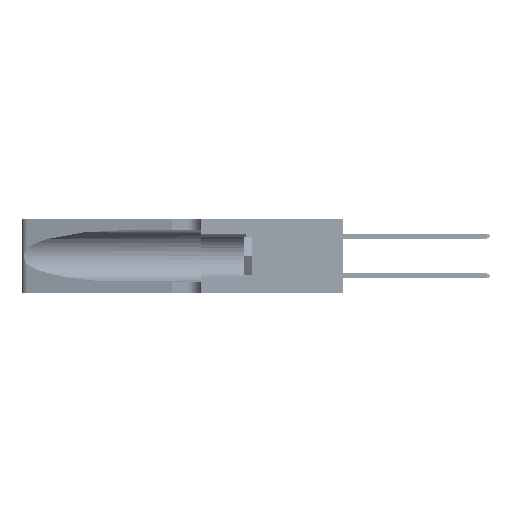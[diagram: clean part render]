
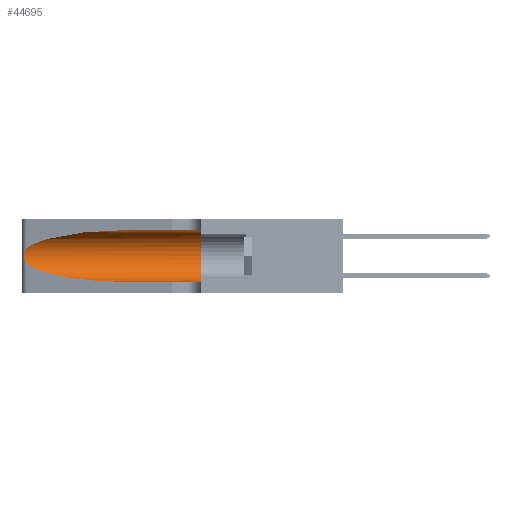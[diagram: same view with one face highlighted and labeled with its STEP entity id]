
A CAD part, left-side view. The second image highlights one B-rep face of the part: STEP entity #44695.
In plain terms, the highlighted cylindrical face has radius 3.308 mm (diameter 6.617 mm), a partial arc.
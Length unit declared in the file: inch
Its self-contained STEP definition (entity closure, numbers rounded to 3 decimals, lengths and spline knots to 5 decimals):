
#1191 = EDGE_CURVE ( 'NONE', #35356, #46719, #9492, .T. ) ;
#1440 = CYLINDRICAL_SURFACE ( 'NONE', #10116, 0.13025 ) ;
#1744 = CARTESIAN_POINT ( 'NONE',  ( 0.25856, 1.23593, 0.16098 ) ) ;
#2813 = FACE_OUTER_BOUND ( 'NONE', #36074, .T. ) ;
#4378 = CARTESIAN_POINT ( 'NONE',  ( 0.1305, 0.72297, 0.05475 ) ) ;
#6072 = ORIENTED_EDGE ( 'NONE', *, *, #26586, .T. ) ;
#6073 = CARTESIAN_POINT ( 'NONE',  ( 0.25639, 1.23186, 0.15144 ) ) ;
#6747 = CARTESIAN_POINT ( 'NONE',  ( 0.2373, 1.15595, 0.28018 ) ) ;
#6760 = B_SPLINE_CURVE_WITH_KNOTS ( 'NONE', 3,
 ( #39694, #10249, #35547, #43905, #18831, #48060, #23069, #52230, #27296, #1744, #31515, #6073, #35724, #10437 ),
 .UNSPECIFIED., .F., .F.,
 ( 4, 2, 2, 2, 2, 2, 4 ),
 ( 0., 0.00027, 0.00053, 0.00107, 0.0016, 0.00187, 0.00214 ),
 .UNSPECIFIED. ) ;
#9492 = LINE ( 'NONE', #49387, #30660 ) ;
#9852 = CARTESIAN_POINT ( 'NONE',  ( 0.1305, 0.72297, 0.05475 ) ) ;
#10116 = AXIS2_PLACEMENT_3D ( 'NONE', #22678, #47687, #30971 ) ;
#10249 = CARTESIAN_POINT ( 'NONE',  ( 0.25555, 1.22994, 0.2215 ) ) ;
#10277 = CIRCLE ( 'NONE', #43381, 0.13025 ) ;
#10437 = CARTESIAN_POINT ( 'NONE',  ( 0.25487, 1.22718, 0.14631 ) ) ;
#11636 = CARTESIAN_POINT ( 'NONE',  ( 0.25487, 1.22718, 0.14631 ) ) ;
#12572 = CARTESIAN_POINT ( 'NONE',  ( 0.1305, 0.35, 0.185 ) ) ;
#13980 = EDGE_CURVE ( 'NONE', #46719, #44644, #10277, .T. ) ;
#14317 = EDGE_CURVE ( 'NONE', #53477, #28655, #6760, .T. ) ;
#16826 = DIRECTION ( 'NONE',  ( 0., 0., 1. ) ) ;
#18767 = EDGE_CURVE ( 'NONE', #35356, #53477, #32263, .T. ) ;
#18831 = CARTESIAN_POINT ( 'NONE',  ( 0.25854, 1.2359, 0.20912 ) ) ;
#19876 = VERTEX_POINT ( 'NONE', #9852 ) ;
#20377 = DIRECTION ( 'NONE',  ( 0., -1., 0. ) ) ;
#21183 = ORIENTED_EDGE ( 'NONE', *, *, #44246, .T. ) ;
#22678 = CARTESIAN_POINT ( 'NONE',  ( 0.1305, 1.61858, 0.185 ) ) ;
#23069 = CARTESIAN_POINT ( 'NONE',  ( 0.26075, 1.23896, 0.19203 ) ) ;
#23721 = CARTESIAN_POINT ( 'NONE',  ( 0.1305, 0.72297, 0.31525 ) ) ;
#25537 = CARTESIAN_POINT ( 'NONE',  ( 0.1305, 0.72297, 0.31525 ) ) ;
#25644 = CARTESIAN_POINT ( 'NONE',  ( 0.25487, 1.22718, 0.14631 ) ) ;
#26586 = EDGE_CURVE ( 'NONE', #28655, #19876, #47555, .T. ) ;
#27296 = CARTESIAN_POINT ( 'NONE',  ( 0.26017, 1.23833, 0.17102 ) ) ;
#27836 = CARTESIAN_POINT ( 'NONE',  ( 0.1305, 0.35, 0.31525 ) ) ;
#28655 = VERTEX_POINT ( 'NONE', #11636 ) ;
#29692 = CARTESIAN_POINT ( 'NONE',  ( 0.2373, 1.15595, 0.08982 ) ) ;
#29859 = CARTESIAN_POINT ( 'NONE',  ( 0.18966, 0.96281, 0.05475 ) ) ;
#30583 = CARTESIAN_POINT ( 'NONE',  ( 0.1305, 0.35, 0.05475 ) ) ;
#30660 = VECTOR ( 'NONE', #20377, 39.37008 ) ;
#30971 = DIRECTION ( 'NONE',  ( 0., 0., -1. ) ) ;
#31515 = CARTESIAN_POINT ( 'NONE',  ( 0.25789, 1.23486, 0.15765 ) ) ;
#32263 =( BOUNDED_CURVE ( )  B_SPLINE_CURVE ( 3, ( #23721, #48692, #6747, #36368 ),
 .UNSPECIFIED., .F., .F. ) 
 B_SPLINE_CURVE_WITH_KNOTS ( ( 4, 4 ),
 ( 1.5708, 2.84003 ),
 .UNSPECIFIED. ) 
 CURVE ( )  GEOMETRIC_REPRESENTATION_ITEM ( )  RATIONAL_B_SPLINE_CURVE ( ( 1., 0.87, 0.87, 1. ) ) 
 REPRESENTATION_ITEM ( '' )  );
#33065 = ORIENTED_EDGE ( 'NONE', *, *, #18767, .T. ) ;
#35356 = VERTEX_POINT ( 'NONE', #25537 ) ;
#35411 = VECTOR ( 'NONE', #41033, 39.37008 ) ;
#35547 = CARTESIAN_POINT ( 'NONE',  ( 0.25639, 1.23184, 0.21858 ) ) ;
#35724 = CARTESIAN_POINT ( 'NONE',  ( 0.25555, 1.22993, 0.14849 ) ) ;
#36074 = EDGE_LOOP ( 'NONE', ( #33065, #36332, #6072, #21183, #38203, #39848 ) ) ;
#36332 = ORIENTED_EDGE ( 'NONE', *, *, #14317, .T. ) ;
#36368 = CARTESIAN_POINT ( 'NONE',  ( 0.25487, 1.22718, 0.22369 ) ) ;
#36729 = LINE ( 'NONE', #36865, #35411 ) ;
#36865 = CARTESIAN_POINT ( 'NONE',  ( 0.1305, 1.61858, 0.05475 ) ) ;
#38203 = ORIENTED_EDGE ( 'NONE', *, *, #13980, .F. ) ;
#39694 = CARTESIAN_POINT ( 'NONE',  ( 0.25487, 1.22718, 0.22369 ) ) ;
#39848 = ORIENTED_EDGE ( 'NONE', *, *, #1191, .F. ) ;
#41033 = DIRECTION ( 'NONE',  ( 0., -1., 0. ) ) ;
#41933 = DIRECTION ( 'NONE',  ( 0., 1., 0. ) ) ;
#43381 = AXIS2_PLACEMENT_3D ( 'NONE', #12572, #41933, #16826 ) ;
#43905 = CARTESIAN_POINT ( 'NONE',  ( 0.25787, 1.23484, 0.2124 ) ) ;
#44246 = EDGE_CURVE ( 'NONE', #19876, #44644, #36729, .T. ) ;
#44644 = VERTEX_POINT ( 'NONE', #30583 ) ;
#44695 = ADVANCED_FACE ( 'NONE', ( #2813 ), #1440, .F. ) ;
#46719 = VERTEX_POINT ( 'NONE', #27836 ) ;
#47555 =( BOUNDED_CURVE ( )  B_SPLINE_CURVE ( 3, ( #25644, #29692, #29859, #4378 ),
 .UNSPECIFIED., .F., .F. ) 
 B_SPLINE_CURVE_WITH_KNOTS ( ( 4, 4 ),
 ( 3.44316, 4.71239 ),
 .UNSPECIFIED. ) 
 CURVE ( )  GEOMETRIC_REPRESENTATION_ITEM ( )  RATIONAL_B_SPLINE_CURVE ( ( 1., 0.87, 0.87, 1. ) ) 
 REPRESENTATION_ITEM ( '' )  );
#47687 = DIRECTION ( 'NONE',  ( 0., -1., 0. ) ) ;
#48060 = CARTESIAN_POINT ( 'NONE',  ( 0.26018, 1.23835, 0.19895 ) ) ;
#48692 = CARTESIAN_POINT ( 'NONE',  ( 0.18966, 0.96281, 0.31525 ) ) ;
#49387 = CARTESIAN_POINT ( 'NONE',  ( 0.1305, 1.61858, 0.31525 ) ) ;
#52230 = CARTESIAN_POINT ( 'NONE',  ( 0.26075, 1.23896, 0.178 ) ) ;
#53145 = CARTESIAN_POINT ( 'NONE',  ( 0.25487, 1.22718, 0.22369 ) ) ;
#53477 = VERTEX_POINT ( 'NONE', #53145 ) ;
